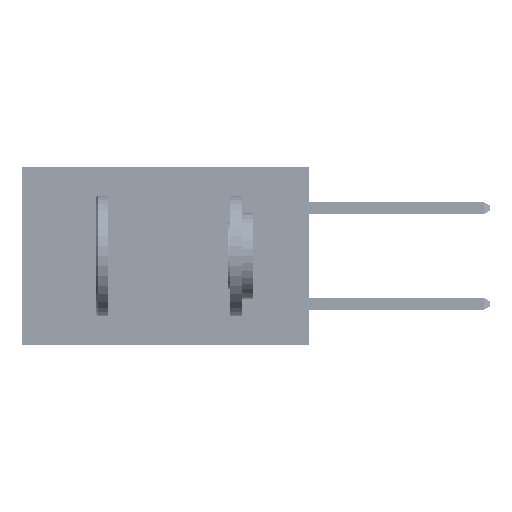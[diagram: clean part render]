
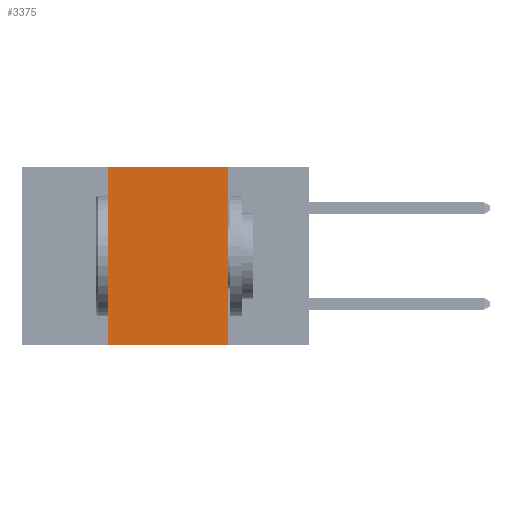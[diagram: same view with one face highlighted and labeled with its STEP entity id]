
A CAD part, left-side view. The second image highlights one B-rep face of the part: STEP entity #3375.
In plain terms, the highlighted planar face has unit normal (-1, 0, 0).
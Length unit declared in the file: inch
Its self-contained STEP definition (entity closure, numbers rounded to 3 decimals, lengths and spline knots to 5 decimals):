
#1160 = LINE ( 'NONE', #35577, #44690 ) ;
#2254 = VERTEX_POINT ( 'NONE', #19618 ) ;
#3375 = ADVANCED_FACE ( 'NONE', ( #9983 ), #7973, .F. ) ;
#6532 = EDGE_LOOP ( 'NONE', ( #30766, #40337, #13153, #40541 ) ) ;
#7973 = PLANE ( 'NONE',  #32736 ) ;
#8647 = VECTOR ( 'NONE', #46504, 39.37008 ) ;
#9813 = VECTOR ( 'NONE', #31946, 39.37008 ) ;
#9983 = FACE_OUTER_BOUND ( 'NONE', #6532, .T. ) ;
#10254 = CARTESIAN_POINT ( 'NONE',  ( 0., 0.6, -0.37 ) ) ;
#10269 = DIRECTION ( 'NONE',  ( 0., 0., -1. ) ) ;
#11595 = VERTEX_POINT ( 'NONE', #28394 ) ;
#11652 = DIRECTION ( 'NONE',  ( 1., 0., 0. ) ) ;
#13153 = ORIENTED_EDGE ( 'NONE', *, *, #26350, .F. ) ;
#19310 = VERTEX_POINT ( 'NONE', #29409 ) ;
#19406 = LINE ( 'NONE', #24894, #8647 ) ;
#19618 = CARTESIAN_POINT ( 'NONE',  ( 0., 0.42, -0.37 ) ) ;
#20581 = LINE ( 'NONE', #10254, #9813 ) ;
#20862 = CARTESIAN_POINT ( 'NONE',  ( 0., 0.42, 0. ) ) ;
#23417 = EDGE_CURVE ( 'NONE', #31522, #11595, #19406, .T. ) ;
#24894 = CARTESIAN_POINT ( 'NONE',  ( 0., 0.6, 0. ) ) ;
#25988 = EDGE_CURVE ( 'NONE', #11595, #19310, #1160, .T. ) ;
#26350 = EDGE_CURVE ( 'NONE', #2254, #31522, #38442, .T. ) ;
#28394 = CARTESIAN_POINT ( 'NONE',  ( 0., 0.17, 0. ) ) ;
#28858 = VECTOR ( 'NONE', #29575, 39.37008 ) ;
#29409 = CARTESIAN_POINT ( 'NONE',  ( 0., 0.17, -0.37 ) ) ;
#29575 = DIRECTION ( 'NONE',  ( 0., 0., 1. ) ) ;
#29700 = CARTESIAN_POINT ( 'NONE',  ( 0., 0.6, 0. ) ) ;
#30766 = ORIENTED_EDGE ( 'NONE', *, *, #25988, .F. ) ;
#31522 = VERTEX_POINT ( 'NONE', #20862 ) ;
#31946 = DIRECTION ( 'NONE',  ( 0., -1., 0. ) ) ;
#32736 = AXIS2_PLACEMENT_3D ( 'NONE', #29700, #11652, #36947 ) ;
#35577 = CARTESIAN_POINT ( 'NONE',  ( 0., 0.17, 0. ) ) ;
#36942 = EDGE_CURVE ( 'NONE', #2254, #19310, #20581, .T. ) ;
#36947 = DIRECTION ( 'NONE',  ( 0., 0., -1. ) ) ;
#38442 = LINE ( 'NONE', #40290, #28858 ) ;
#40290 = CARTESIAN_POINT ( 'NONE',  ( 0., 0.42, 0. ) ) ;
#40337 = ORIENTED_EDGE ( 'NONE', *, *, #23417, .F. ) ;
#40541 = ORIENTED_EDGE ( 'NONE', *, *, #36942, .T. ) ;
#44690 = VECTOR ( 'NONE', #10269, 39.37008 ) ;
#46504 = DIRECTION ( 'NONE',  ( 0., -1., 0. ) ) ;
